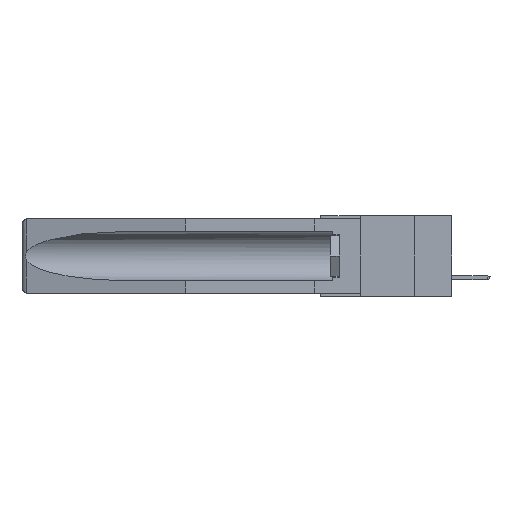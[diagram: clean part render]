
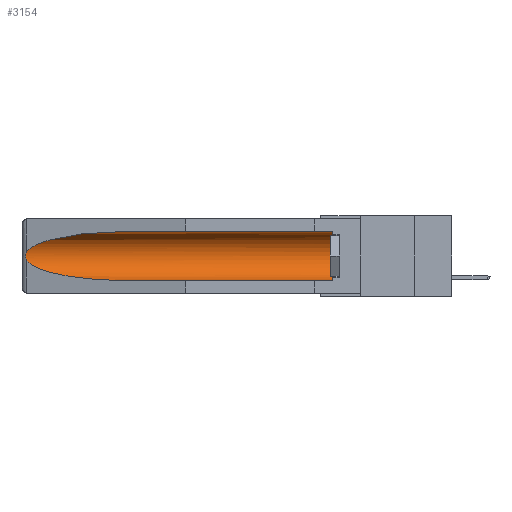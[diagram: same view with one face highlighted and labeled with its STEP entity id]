
A CAD part, left-side view. The second image highlights one B-rep face of the part: STEP entity #3154.
In plain terms, the highlighted cylindrical face has radius 2.857 mm (diameter 5.715 mm), a partial arc.
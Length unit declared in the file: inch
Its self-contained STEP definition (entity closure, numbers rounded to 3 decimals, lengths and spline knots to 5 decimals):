
#446 = DIRECTION ( 'NONE',  ( 0., 1., 0. ) ) ;
#749 = ORIENTED_EDGE ( 'NONE', *, *, #23529, .T. ) ;
#1076 = ORIENTED_EDGE ( 'NONE', *, *, #11915, .T. ) ;
#1343 = CARTESIAN_POINT ( 'NONE',  ( 0.155, -0.30754, -0.284 ) ) ;
#1344 = DIRECTION ( 'NONE',  ( 0., 0., 1. ) ) ;
#1909 = CARTESIAN_POINT ( 'NONE',  ( 0.2673, 1.53269, -0.17917 ) ) ;
#2727 = LINE ( 'NONE', #1343, #23863 ) ;
#2975 = DIRECTION ( 'NONE',  ( 0., 1., 0. ) ) ;
#3058 = DIRECTION ( 'NONE',  ( 0., -1., 0. ) ) ;
#3099 = VERTEX_POINT ( 'NONE', #20269 ) ;
#3154 = ADVANCED_FACE ( 'NONE', ( #18034 ), #19569, .F. ) ;
#3648 = CARTESIAN_POINT ( 'NONE',  ( 0.25451, 1.48313, -0.09465 ) ) ;
#3698 = CARTESIAN_POINT ( 'NONE',  ( 0.2675, 1.53308, -0.17534 ) ) ;
#4675 = ORIENTED_EDGE ( 'NONE', *, *, #13069, .F. ) ;
#4837 = ORIENTED_EDGE ( 'NONE', *, *, #12472, .T. ) ;
#5431 = VERTEX_POINT ( 'NONE', #18764 ) ;
#5533 = CARTESIAN_POINT ( 'NONE',  ( 0.155, 1.07973, -0.059 ) ) ;
#6254 = CARTESIAN_POINT ( 'NONE',  ( 0.155, -0.30754, -0.059 ) ) ;
#6723 =( BOUNDED_CURVE ( )  B_SPLINE_CURVE ( 3, ( #12717, #14388, #8757, #16497 ),
 .UNSPECIFIED., .F., .F. ) 
 B_SPLINE_CURVE_WITH_KNOTS ( ( 4, 4 ),
 ( 0.1948, 1.5708 ),
 .UNSPECIFIED. ) 
 CURVE ( )  GEOMETRIC_REPRESENTATION_ITEM ( )  RATIONAL_B_SPLINE_CURVE ( ( 1., 0.848, 0.848, 1. ) ) 
 REPRESENTATION_ITEM ( '' )  );
#7052 = CARTESIAN_POINT ( 'NONE',  ( 0.155, 1.07973, -0.284 ) ) ;
#7419 = CARTESIAN_POINT ( 'NONE',  ( 0.21114, 1.30732, -0.059 ) ) ;
#7465 = CARTESIAN_POINT ( 'NONE',  ( 0.2675, 1.53308, -0.16763 ) ) ;
#7794 = CARTESIAN_POINT ( 'NONE',  ( 0.26655, 1.53094, -0.18657 ) ) ;
#7917 = B_SPLINE_CURVE_WITH_KNOTS ( 'NONE', 3,
 ( #15461, #17263, #19460, #19381, #7465, #3698, #1909, #7794, #13496, #13410 ),
 .UNSPECIFIED., .F., .F.,
 ( 4, 2, 2, 2, 4 ),
 ( 0., 0.00029, 0.00058, 0.00087, 0.00117 ),
 .UNSPECIFIED. ) ;
#8483 = LINE ( 'NONE', #6254, #24684 ) ;
#8757 = CARTESIAN_POINT ( 'NONE',  ( 0.21114, 1.30732, -0.284 ) ) ;
#8921 = CARTESIAN_POINT ( 'NONE',  ( 0.155, 0.126, -0.059 ) ) ;
#9223 = CARTESIAN_POINT ( 'NONE',  ( 0.155, 0.126, -0.1715 ) ) ;
#9560 = CARTESIAN_POINT ( 'NONE',  ( 0.26537, 1.52718, -0.19328 ) ) ;
#10318 = CARTESIAN_POINT ( 'NONE',  ( 0.155, 0.126, -0.284 ) ) ;
#10482 = EDGE_CURVE ( 'NONE', #3099, #5431, #12494, .T. ) ;
#11553 = VERTEX_POINT ( 'NONE', #10318 ) ;
#11915 = EDGE_CURVE ( 'NONE', #5431, #20477, #7917, .T. ) ;
#12472 = EDGE_CURVE ( 'NONE', #11553, #17360, #23600, .T. ) ;
#12494 =( BOUNDED_CURVE ( )  B_SPLINE_CURVE ( 3, ( #5533, #7419, #3648, #19322 ),
 .UNSPECIFIED., .F., .F. ) 
 B_SPLINE_CURVE_WITH_KNOTS ( ( 4, 4 ),
 ( 4.71239, 6.08839 ),
 .UNSPECIFIED. ) 
 CURVE ( )  GEOMETRIC_REPRESENTATION_ITEM ( )  RATIONAL_B_SPLINE_CURVE ( ( 1., 0.848, 0.848, 1. ) ) 
 REPRESENTATION_ITEM ( '' )  );
#12668 = CARTESIAN_POINT ( 'NONE',  ( 0.155, -0.30754, -0.1715 ) ) ;
#12717 = CARTESIAN_POINT ( 'NONE',  ( 0.26537, 1.52718, -0.19328 ) ) ;
#12997 = DIRECTION ( 'NONE',  ( 0., 1., 0. ) ) ;
#13069 = EDGE_CURVE ( 'NONE', #11553, #24284, #2727, .T. ) ;
#13410 = CARTESIAN_POINT ( 'NONE',  ( 0.26537, 1.52718, -0.19328 ) ) ;
#13496 = CARTESIAN_POINT ( 'NONE',  ( 0.26597, 1.5296, -0.19026 ) ) ;
#13853 = ORIENTED_EDGE ( 'NONE', *, *, #10482, .T. ) ;
#14388 = CARTESIAN_POINT ( 'NONE',  ( 0.25451, 1.48313, -0.24835 ) ) ;
#14742 = DIRECTION ( 'NONE',  ( 0., 0., 1. ) ) ;
#15461 = CARTESIAN_POINT ( 'NONE',  ( 0.26537, 1.52718, -0.14972 ) ) ;
#15908 = ORIENTED_EDGE ( 'NONE', *, *, #24794, .T. ) ;
#16497 = CARTESIAN_POINT ( 'NONE',  ( 0.155, 1.07973, -0.284 ) ) ;
#16545 = EDGE_LOOP ( 'NONE', ( #13853, #1076, #749, #4675, #4837, #15908 ) ) ;
#16750 = AXIS2_PLACEMENT_3D ( 'NONE', #9223, #3058, #1344 ) ;
#17263 = CARTESIAN_POINT ( 'NONE',  ( 0.26597, 1.52961, -0.15275 ) ) ;
#17360 = VERTEX_POINT ( 'NONE', #8921 ) ;
#18034 = FACE_OUTER_BOUND ( 'NONE', #16545, .T. ) ;
#18764 = CARTESIAN_POINT ( 'NONE',  ( 0.26537, 1.52718, -0.14972 ) ) ;
#19322 = CARTESIAN_POINT ( 'NONE',  ( 0.26537, 1.52718, -0.14972 ) ) ;
#19381 = CARTESIAN_POINT ( 'NONE',  ( 0.2673, 1.5327, -0.16383 ) ) ;
#19460 = CARTESIAN_POINT ( 'NONE',  ( 0.26654, 1.53092, -0.15636 ) ) ;
#19569 = CYLINDRICAL_SURFACE ( 'NONE', #21323, 0.1125 ) ;
#20269 = CARTESIAN_POINT ( 'NONE',  ( 0.155, 1.07973, -0.059 ) ) ;
#20477 = VERTEX_POINT ( 'NONE', #9560 ) ;
#21323 = AXIS2_PLACEMENT_3D ( 'NONE', #12668, #2975, #14742 ) ;
#23529 = EDGE_CURVE ( 'NONE', #20477, #24284, #6723, .T. ) ;
#23600 = CIRCLE ( 'NONE', #16750, 0.1125 ) ;
#23863 = VECTOR ( 'NONE', #12997, 39.37008 ) ;
#24284 = VERTEX_POINT ( 'NONE', #7052 ) ;
#24684 = VECTOR ( 'NONE', #446, 39.37008 ) ;
#24794 = EDGE_CURVE ( 'NONE', #17360, #3099, #8483, .T. ) ;
